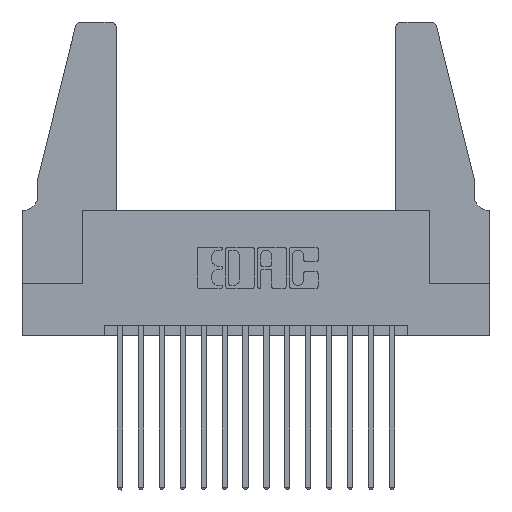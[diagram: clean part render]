
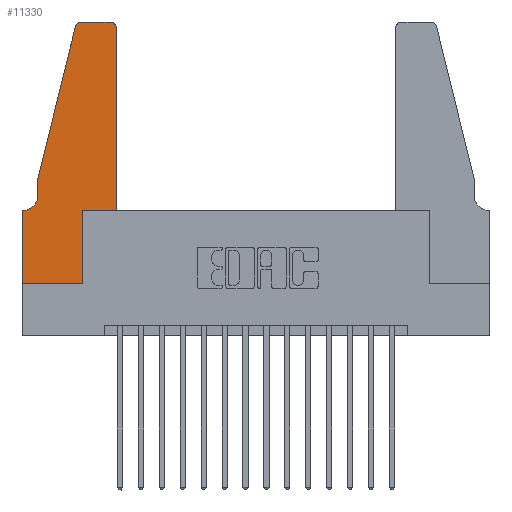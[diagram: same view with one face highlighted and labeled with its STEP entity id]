
A CAD part, top view. The second image highlights one B-rep face of the part: STEP entity #11330.
In plain terms, the highlighted planar face has unit normal (0, 0, 1).
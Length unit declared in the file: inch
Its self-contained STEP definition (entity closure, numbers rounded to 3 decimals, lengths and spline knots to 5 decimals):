
#44 = VERTEX_POINT ( 'NONE', #15220 ) ;
#355 = VERTEX_POINT ( 'NONE', #11911 ) ;
#603 = LINE ( 'NONE', #16180, #11479 ) ;
#609 = DIRECTION ( 'NONE',  ( 0., 1., 0. ) ) ;
#642 = LINE ( 'NONE', #3828, #7153 ) ;
#964 = VERTEX_POINT ( 'NONE', #1648 ) ;
#1007 = VERTEX_POINT ( 'NONE', #9683 ) ;
#1032 = DIRECTION ( 'NONE',  ( 0., -1., 0. ) ) ;
#1494 = DIRECTION ( 'NONE',  ( 1., 0., 0. ) ) ;
#1545 = VERTEX_POINT ( 'NONE', #6431 ) ;
#1580 = DIRECTION ( 'NONE',  ( 0., 0., 1. ) ) ;
#1648 = CARTESIAN_POINT ( 'NONE',  ( 0.4505, 0.35, 0.37 ) ) ;
#2313 = VERTEX_POINT ( 'NONE', #4782 ) ;
#2759 = DIRECTION ( 'NONE',  ( -1., 0., 0. ) ) ;
#2808 = ORIENTED_EDGE ( 'NONE', *, *, #8017, .T. ) ;
#3202 = VECTOR ( 'NONE', #8722, 39.37008 ) ;
#3532 = CARTESIAN_POINT ( 'NONE',  ( 0.284, 1.25, 0.37 ) ) ;
#3621 = LINE ( 'NONE', #7401, #3202 ) ;
#3682 = ORIENTED_EDGE ( 'NONE', *, *, #14755, .T. ) ;
#3775 = VECTOR ( 'NONE', #14153, 39.37008 ) ;
#3828 = CARTESIAN_POINT ( 'NONE',  ( 0.0755, 0.5, 0.37 ) ) ;
#4083 = LINE ( 'NONE', #16771, #9391 ) ;
#4202 = EDGE_CURVE ( 'NONE', #1007, #44, #11193, .T. ) ;
#4382 = VECTOR ( 'NONE', #14636, 39.37008 ) ;
#4542 = EDGE_CURVE ( 'NONE', #5101, #1545, #7847, .T. ) ;
#4663 = EDGE_CURVE ( 'NONE', #10916, #8739, #14259, .T. ) ;
#4782 = CARTESIAN_POINT ( 'NONE',  ( 0.0055, 0.35, 0.37 ) ) ;
#4816 = ORIENTED_EDGE ( 'NONE', *, *, #10997, .T. ) ;
#4872 = CARTESIAN_POINT ( 'NONE',  ( 0.4205, 1.22, 0.37 ) ) ;
#5044 = DIRECTION ( 'NONE',  ( 0., 0., 1. ) ) ;
#5101 = VERTEX_POINT ( 'NONE', #12848 ) ;
#5113 = DIRECTION ( 'NONE',  ( 0., 0., -1. ) ) ;
#5943 = EDGE_CURVE ( 'NONE', #8739, #2313, #13165, .T. ) ;
#6027 = VERTEX_POINT ( 'NONE', #16251 ) ;
#6085 = CARTESIAN_POINT ( 'NONE',  ( 0.2605, 1.25, 0.37 ) ) ;
#6235 = VECTOR ( 'NONE', #13043, 39.37008 ) ;
#6344 = DIRECTION ( 'NONE',  ( 1., 0., 0. ) ) ;
#6429 = ORIENTED_EDGE ( 'NONE', *, *, #4202, .T. ) ;
#6431 = CARTESIAN_POINT ( 'NONE',  ( 0.2865, 0., 0.37 ) ) ;
#6432 = AXIS2_PLACEMENT_3D ( 'NONE', #4872, #5044, #6344 ) ;
#6719 = LINE ( 'NONE', #6085, #11706 ) ;
#6857 = AXIS2_PLACEMENT_3D ( 'NONE', #10807, #1580, #9223 ) ;
#7153 = VECTOR ( 'NONE', #10437, 39.37008 ) ;
#7401 = CARTESIAN_POINT ( 'NONE',  ( 0.4505, 0.35, 0.37 ) ) ;
#7510 = CARTESIAN_POINT ( 'NONE',  ( 0.0755, 0.5, 0.37 ) ) ;
#7540 = ORIENTED_EDGE ( 'NONE', *, *, #8282, .T. ) ;
#7745 = EDGE_CURVE ( 'NONE', #6027, #10916, #642, .T. ) ;
#7847 = LINE ( 'NONE', #9997, #3775 ) ;
#7910 = VECTOR ( 'NONE', #2759, 39.37008 ) ;
#8017 = EDGE_CURVE ( 'NONE', #355, #5101, #4083, .T. ) ;
#8030 = CARTESIAN_POINT ( 'NONE',  ( 0., 0.35, 0.37 ) ) ;
#8282 = EDGE_CURVE ( 'NONE', #1545, #15618, #603, .T. ) ;
#8597 = AXIS2_PLACEMENT_3D ( 'NONE', #8030, #14657, #1494 ) ;
#8722 = DIRECTION ( 'NONE',  ( 0., 1., 0. ) ) ;
#8739 = VERTEX_POINT ( 'NONE', #10599 ) ;
#8894 = VERTEX_POINT ( 'NONE', #3532 ) ;
#9223 = DIRECTION ( 'NONE',  ( 1., 0., 0. ) ) ;
#9241 = DIRECTION ( 'NONE',  ( -1., 0., 0. ) ) ;
#9391 = VECTOR ( 'NONE', #1032, 39.37008 ) ;
#9683 = CARTESIAN_POINT ( 'NONE',  ( 0.4505, 1.22, 0.37 ) ) ;
#9754 = LINE ( 'NONE', #14383, #6235 ) ;
#9997 = CARTESIAN_POINT ( 'NONE',  ( 0., 0., 0.37 ) ) ;
#10258 = ORIENTED_EDGE ( 'NONE', *, *, #7745, .T. ) ;
#10437 = DIRECTION ( 'NONE',  ( -0.239, -0.971, 0. ) ) ;
#10599 = CARTESIAN_POINT ( 'NONE',  ( 0.0755, 0.42, 0.37 ) ) ;
#10762 = EDGE_CURVE ( 'NONE', #964, #1007, #3621, .T. ) ;
#10807 = CARTESIAN_POINT ( 'NONE',  ( 0.284, 1.22, 0.37 ) ) ;
#10916 = VERTEX_POINT ( 'NONE', #7510 ) ;
#10997 = EDGE_CURVE ( 'NONE', #15618, #964, #9754, .T. ) ;
#11001 = AXIS2_PLACEMENT_3D ( 'NONE', #15509, #5113, #9241 ) ;
#11193 = CIRCLE ( 'NONE', #6432, 0.03 ) ;
#11330 = ADVANCED_FACE ( 'NONE', ( #13042 ), #15904, .T. ) ;
#11463 = LINE ( 'NONE', #12980, #7910 ) ;
#11479 = VECTOR ( 'NONE', #609, 39.37008 ) ;
#11706 = VECTOR ( 'NONE', #15303, 39.37008 ) ;
#11911 = CARTESIAN_POINT ( 'NONE',  ( 0., 0.35, 0.37 ) ) ;
#11962 = CARTESIAN_POINT ( 'NONE',  ( 0.0755, 0.5, 0.37 ) ) ;
#12314 = ORIENTED_EDGE ( 'NONE', *, *, #4663, .T. ) ;
#12848 = CARTESIAN_POINT ( 'NONE',  ( 0., 0., 0.37 ) ) ;
#12980 = CARTESIAN_POINT ( 'NONE',  ( 0.0755, 0.35, 0.37 ) ) ;
#13042 = FACE_OUTER_BOUND ( 'NONE', #16750, .T. ) ;
#13043 = DIRECTION ( 'NONE',  ( 1., 0., 0. ) ) ;
#13056 = ORIENTED_EDGE ( 'NONE', *, *, #16674, .T. ) ;
#13165 = CIRCLE ( 'NONE', #11001, 0.07 ) ;
#13172 = ORIENTED_EDGE ( 'NONE', *, *, #15177, .T. ) ;
#13276 = ORIENTED_EDGE ( 'NONE', *, *, #4542, .T. ) ;
#13762 = CIRCLE ( 'NONE', #6857, 0.03 ) ;
#14153 = DIRECTION ( 'NONE',  ( 1., 0., 0. ) ) ;
#14259 = LINE ( 'NONE', #11962, #4382 ) ;
#14383 = CARTESIAN_POINT ( 'NONE',  ( 0.4505, 0.35, 0.37 ) ) ;
#14636 = DIRECTION ( 'NONE',  ( 0., -1., 0. ) ) ;
#14657 = DIRECTION ( 'NONE',  ( 0., 0., 1. ) ) ;
#14755 = EDGE_CURVE ( 'NONE', #8894, #6027, #13762, .T. ) ;
#14906 = ORIENTED_EDGE ( 'NONE', *, *, #10762, .T. ) ;
#15177 = EDGE_CURVE ( 'NONE', #44, #8894, #6719, .T. ) ;
#15220 = CARTESIAN_POINT ( 'NONE',  ( 0.4205, 1.25, 0.37 ) ) ;
#15303 = DIRECTION ( 'NONE',  ( -1., 0., 0. ) ) ;
#15509 = CARTESIAN_POINT ( 'NONE',  ( 0.0055, 0.42, 0.37 ) ) ;
#15618 = VERTEX_POINT ( 'NONE', #16380 ) ;
#15904 = PLANE ( 'NONE',  #8597 ) ;
#16046 = ORIENTED_EDGE ( 'NONE', *, *, #5943, .T. ) ;
#16180 = CARTESIAN_POINT ( 'NONE',  ( 0.2865, 0.35, 0.37 ) ) ;
#16251 = CARTESIAN_POINT ( 'NONE',  ( 0.25487, 1.22718, 0.37 ) ) ;
#16380 = CARTESIAN_POINT ( 'NONE',  ( 0.2865, 0.35, 0.37 ) ) ;
#16674 = EDGE_CURVE ( 'NONE', #2313, #355, #11463, .T. ) ;
#16750 = EDGE_LOOP ( 'NONE', ( #13172, #3682, #10258, #12314, #16046, #13056, #2808, #13276, #7540, #4816, #14906, #6429 ) ) ;
#16771 = CARTESIAN_POINT ( 'NONE',  ( 0., 0., 0.37 ) ) ;
